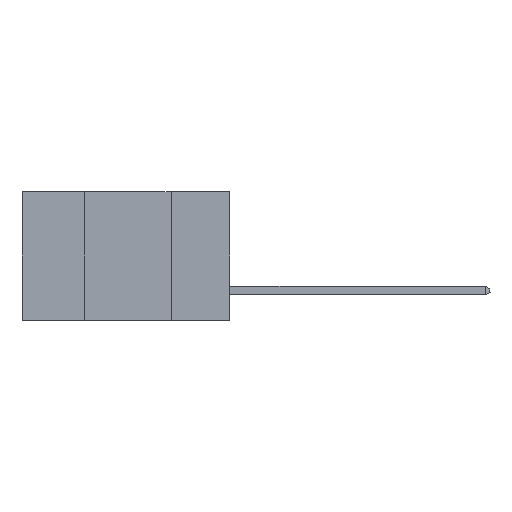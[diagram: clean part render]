
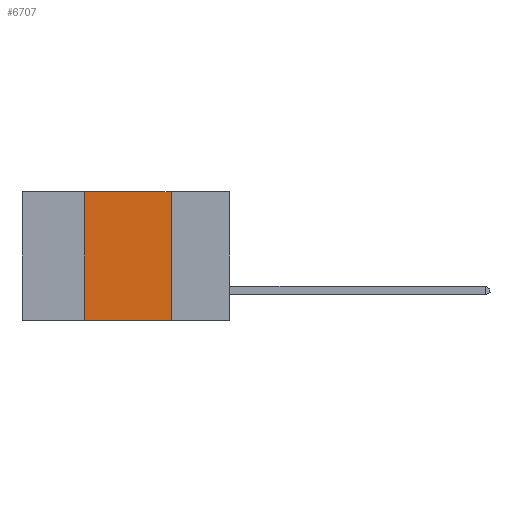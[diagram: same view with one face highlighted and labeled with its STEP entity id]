
A CAD part, left-side view. The second image highlights one B-rep face of the part: STEP entity #6707.
In plain terms, the highlighted planar face has unit normal (-1, 0, 0).
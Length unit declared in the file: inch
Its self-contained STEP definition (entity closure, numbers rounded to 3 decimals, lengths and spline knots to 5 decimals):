
#1446 = VECTOR ( 'NONE', #7535, 39.37008 ) ;
#1449 = DIRECTION ( 'NONE',  ( 0., -1., 0. ) ) ;
#1595 = ORIENTED_EDGE ( 'NONE', *, *, #7188, .F. ) ;
#1928 = VERTEX_POINT ( 'NONE', #6366 ) ;
#2333 = PLANE ( 'NONE',  #4306 ) ;
#2397 = DIRECTION ( 'NONE',  ( 1., 0., 0. ) ) ;
#2404 = CARTESIAN_POINT ( 'NONE',  ( 0., 0.17, -0.37 ) ) ;
#3075 = LINE ( 'NONE', #8970, #3669 ) ;
#3101 = DIRECTION ( 'NONE',  ( 0., 0., -1. ) ) ;
#3107 = VERTEX_POINT ( 'NONE', #3925 ) ;
#3669 = VECTOR ( 'NONE', #1449, 39.37008 ) ;
#3925 = CARTESIAN_POINT ( 'NONE',  ( 0., 0.42, 0. ) ) ;
#4045 = EDGE_CURVE ( 'NONE', #3107, #1928, #3075, .T. ) ;
#4306 = AXIS2_PLACEMENT_3D ( 'NONE', #6899, #2397, #3101 ) ;
#5020 = CARTESIAN_POINT ( 'NONE',  ( 0., 0.17, 0. ) ) ;
#5460 = FACE_OUTER_BOUND ( 'NONE', #7763, .T. ) ;
#5478 = ORIENTED_EDGE ( 'NONE', *, *, #7835, .T. ) ;
#5901 = CARTESIAN_POINT ( 'NONE',  ( 0., 0.42, -0.37 ) ) ;
#6366 = CARTESIAN_POINT ( 'NONE',  ( 0., 0.17, 0. ) ) ;
#6460 = DIRECTION ( 'NONE',  ( 0., 0., -1. ) ) ;
#6469 = ORIENTED_EDGE ( 'NONE', *, *, #4045, .F. ) ;
#6707 = ADVANCED_FACE ( 'NONE', ( #5460 ), #2333, .F. ) ;
#6899 = CARTESIAN_POINT ( 'NONE',  ( 0., 0.6, 0. ) ) ;
#7188 = EDGE_CURVE ( 'NONE', #7641, #3107, #9417, .T. ) ;
#7299 = VECTOR ( 'NONE', #6460, 39.37008 ) ;
#7443 = VECTOR ( 'NONE', #9092, 39.37008 ) ;
#7535 = DIRECTION ( 'NONE',  ( 0., -1., 0. ) ) ;
#7545 = LINE ( 'NONE', #8892, #1446 ) ;
#7641 = VERTEX_POINT ( 'NONE', #5901 ) ;
#7763 = EDGE_LOOP ( 'NONE', ( #7878, #6469, #1595, #5478 ) ) ;
#7835 = EDGE_CURVE ( 'NONE', #7641, #9045, #7545, .T. ) ;
#7878 = ORIENTED_EDGE ( 'NONE', *, *, #8186, .F. ) ;
#8186 = EDGE_CURVE ( 'NONE', #1928, #9045, #8931, .T. ) ;
#8892 = CARTESIAN_POINT ( 'NONE',  ( 0., 0.6, -0.37 ) ) ;
#8931 = LINE ( 'NONE', #5020, #7299 ) ;
#8970 = CARTESIAN_POINT ( 'NONE',  ( 0., 0.6, 0. ) ) ;
#9028 = CARTESIAN_POINT ( 'NONE',  ( 0., 0.42, 0. ) ) ;
#9045 = VERTEX_POINT ( 'NONE', #2404 ) ;
#9092 = DIRECTION ( 'NONE',  ( 0., 0., 1. ) ) ;
#9417 = LINE ( 'NONE', #9028, #7443 ) ;
